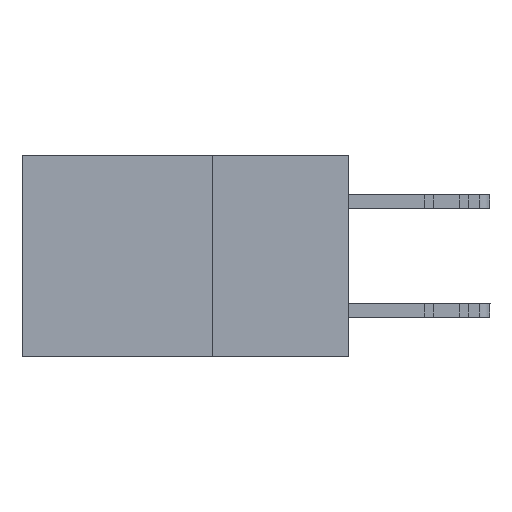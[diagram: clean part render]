
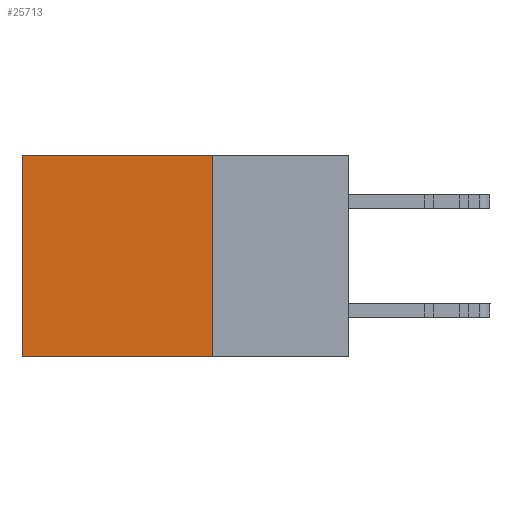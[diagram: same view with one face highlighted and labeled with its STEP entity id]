
A CAD part, left-side view. The second image highlights one B-rep face of the part: STEP entity #25713.
In plain terms, the highlighted planar face has unit normal (-1, 0, 0).
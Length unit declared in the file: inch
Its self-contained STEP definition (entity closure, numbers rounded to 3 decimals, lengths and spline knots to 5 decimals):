
#529 = EDGE_CURVE ( 'NONE', #23503, #11611, #19030, .T. ) ;
#641 = ORIENTED_EDGE ( 'NONE', *, *, #529, .F. ) ;
#1543 = VECTOR ( 'NONE', #10258, 39.37008 ) ;
#2336 = VECTOR ( 'NONE', #13782, 39.37008 ) ;
#2364 = DIRECTION ( 'NONE',  ( 0., 0., -1. ) ) ;
#2526 = VERTEX_POINT ( 'NONE', #23241 ) ;
#4059 = DIRECTION ( 'NONE',  ( 0., 1., 0. ) ) ;
#7199 = ORIENTED_EDGE ( 'NONE', *, *, #15943, .T. ) ;
#7619 = PLANE ( 'NONE',  #7639 ) ;
#7639 = AXIS2_PLACEMENT_3D ( 'NONE', #17966, #26490, #13899 ) ;
#10258 = DIRECTION ( 'NONE',  ( 0., 1., 0. ) ) ;
#10329 = EDGE_CURVE ( 'NONE', #11611, #2526, #12615, .T. ) ;
#11407 = ORIENTED_EDGE ( 'NONE', *, *, #10329, .F. ) ;
#11611 = VERTEX_POINT ( 'NONE', #20871 ) ;
#11673 = EDGE_CURVE ( 'NONE', #13512, #2526, #24117, .T. ) ;
#12077 = CARTESIAN_POINT ( 'NONE',  ( 0.2615, 0.25, 0. ) ) ;
#12615 = LINE ( 'NONE', #18700, #18202 ) ;
#13133 = EDGE_LOOP ( 'NONE', ( #17774, #11407, #641, #7199 ) ) ;
#13201 = FACE_OUTER_BOUND ( 'NONE', #13133, .T. ) ;
#13512 = VERTEX_POINT ( 'NONE', #24756 ) ;
#13782 = DIRECTION ( 'NONE',  ( 0., 0., -1. ) ) ;
#13899 = DIRECTION ( 'NONE',  ( 0., 0., -1. ) ) ;
#14335 = CARTESIAN_POINT ( 'NONE',  ( 0.2615, 0.25, -0.37 ) ) ;
#15943 = EDGE_CURVE ( 'NONE', #23503, #13512, #18248, .T. ) ;
#17774 = ORIENTED_EDGE ( 'NONE', *, *, #11673, .T. ) ;
#17840 = VECTOR ( 'NONE', #2364, 39.37008 ) ;
#17966 = CARTESIAN_POINT ( 'NONE',  ( 0.2615, 0.25, -0.37 ) ) ;
#18202 = VECTOR ( 'NONE', #4059, 39.37008 ) ;
#18248 = LINE ( 'NONE', #24954, #1543 ) ;
#18700 = CARTESIAN_POINT ( 'NONE',  ( 0.2615, 0.25, -0.37 ) ) ;
#19030 = LINE ( 'NONE', #14335, #2336 ) ;
#20871 = CARTESIAN_POINT ( 'NONE',  ( 0.2615, 0.25, -0.37 ) ) ;
#21128 = CARTESIAN_POINT ( 'NONE',  ( 0.2615, 0.6, -0.37 ) ) ;
#23241 = CARTESIAN_POINT ( 'NONE',  ( 0.2615, 0.6, -0.37 ) ) ;
#23503 = VERTEX_POINT ( 'NONE', #12077 ) ;
#24117 = LINE ( 'NONE', #21128, #17840 ) ;
#24756 = CARTESIAN_POINT ( 'NONE',  ( 0.2615, 0.6, 0. ) ) ;
#24954 = CARTESIAN_POINT ( 'NONE',  ( 0.2615, 0.25, 0. ) ) ;
#25713 = ADVANCED_FACE ( 'NONE', ( #13201 ), #7619, .F. ) ;
#26490 = DIRECTION ( 'NONE',  ( 1., 0., 0. ) ) ;
